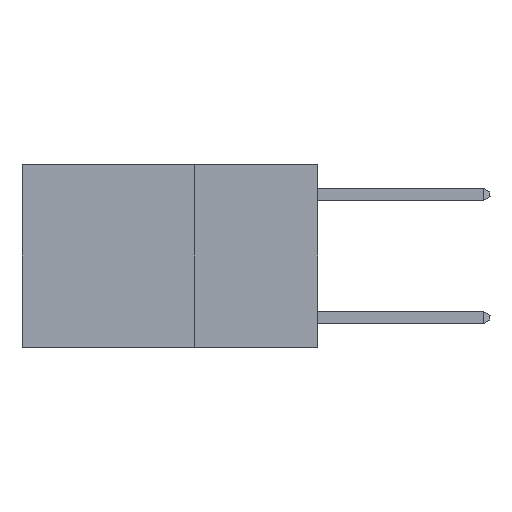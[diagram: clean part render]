
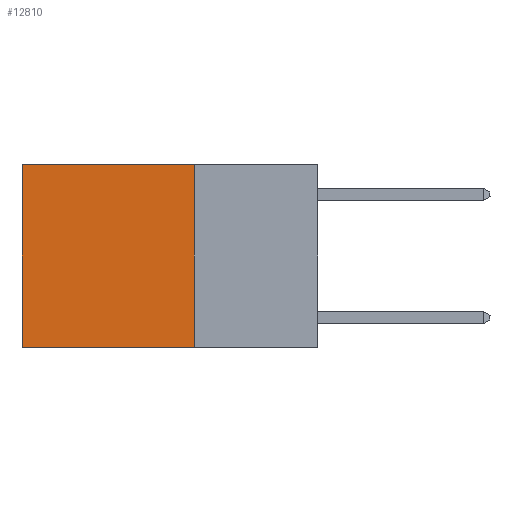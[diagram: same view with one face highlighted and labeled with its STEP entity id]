
A CAD part, left-side view. The second image highlights one B-rep face of the part: STEP entity #12810.
In plain terms, the highlighted planar face has unit normal (-1, 0, 0).
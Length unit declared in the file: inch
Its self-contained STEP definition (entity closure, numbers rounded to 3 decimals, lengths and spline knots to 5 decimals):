
#599 = CARTESIAN_POINT ( 'NONE',  ( 0.2625, 0.25, 0. ) ) ;
#880 = CARTESIAN_POINT ( 'NONE',  ( 0.2625, 0.25, 0. ) ) ;
#1434 = ORIENTED_EDGE ( 'NONE', *, *, #9148, .F. ) ;
#2674 = AXIS2_PLACEMENT_3D ( 'NONE', #4686, #12044, #4767 ) ;
#2850 = DIRECTION ( 'NONE',  ( 0., 1., 0. ) ) ;
#2994 = VERTEX_POINT ( 'NONE', #3378 ) ;
#3042 = DIRECTION ( 'NONE',  ( 0., 0., -1. ) ) ;
#3378 = CARTESIAN_POINT ( 'NONE',  ( 0.2625, 0.25, -0.37 ) ) ;
#4145 = VECTOR ( 'NONE', #3042, 39.37008 ) ;
#4472 = EDGE_CURVE ( 'NONE', #10046, #13040, #5692, .T. ) ;
#4686 = CARTESIAN_POINT ( 'NONE',  ( 0.2625, 0.25, 0. ) ) ;
#4767 = DIRECTION ( 'NONE',  ( 0., 0., -1. ) ) ;
#5686 = DIRECTION ( 'NONE',  ( 0., 0., -1. ) ) ;
#5692 = LINE ( 'NONE', #880, #12301 ) ;
#5888 = ORIENTED_EDGE ( 'NONE', *, *, #13772, .T. ) ;
#6412 = CARTESIAN_POINT ( 'NONE',  ( 0.2625, 0.6, 0. ) ) ;
#6657 = CARTESIAN_POINT ( 'NONE',  ( 0.2625, 0.25, 0. ) ) ;
#7066 = FACE_OUTER_BOUND ( 'NONE', #10661, .T. ) ;
#7739 = ORIENTED_EDGE ( 'NONE', *, *, #4472, .T. ) ;
#8206 = VERTEX_POINT ( 'NONE', #9729 ) ;
#8362 = PLANE ( 'NONE',  #2674 ) ;
#8403 = DIRECTION ( 'NONE',  ( 0., 1., 0. ) ) ;
#9148 = EDGE_CURVE ( 'NONE', #10046, #2994, #13567, .T. ) ;
#9515 = VECTOR ( 'NONE', #5686, 39.37008 ) ;
#9729 = CARTESIAN_POINT ( 'NONE',  ( 0.2625, 0.6, -0.37 ) ) ;
#9826 = LINE ( 'NONE', #13615, #10561 ) ;
#10046 = VERTEX_POINT ( 'NONE', #599 ) ;
#10561 = VECTOR ( 'NONE', #2850, 39.37008 ) ;
#10661 = EDGE_LOOP ( 'NONE', ( #5888, #11870, #1434, #7739 ) ) ;
#10977 = CARTESIAN_POINT ( 'NONE',  ( 0.2625, 0.6, 0. ) ) ;
#11870 = ORIENTED_EDGE ( 'NONE', *, *, #14922, .F. ) ;
#12044 = DIRECTION ( 'NONE',  ( 1., 0., 0. ) ) ;
#12301 = VECTOR ( 'NONE', #8403, 39.37008 ) ;
#12810 = ADVANCED_FACE ( 'NONE', ( #7066 ), #8362, .F. ) ;
#13040 = VERTEX_POINT ( 'NONE', #6412 ) ;
#13567 = LINE ( 'NONE', #6657, #4145 ) ;
#13615 = CARTESIAN_POINT ( 'NONE',  ( 0.2625, 0.25, -0.37 ) ) ;
#13772 = EDGE_CURVE ( 'NONE', #13040, #8206, #15360, .T. ) ;
#14922 = EDGE_CURVE ( 'NONE', #2994, #8206, #9826, .T. ) ;
#15360 = LINE ( 'NONE', #10977, #9515 ) ;
